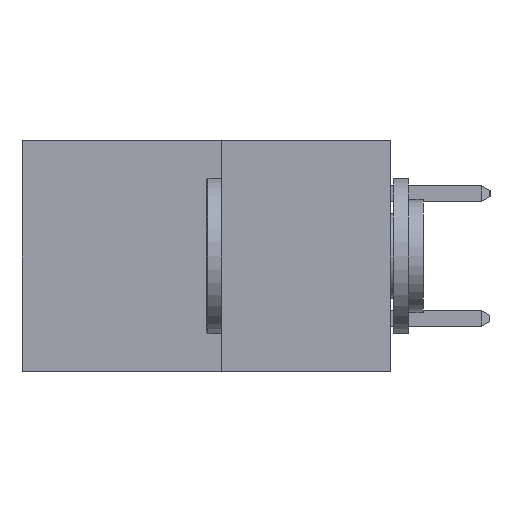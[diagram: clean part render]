
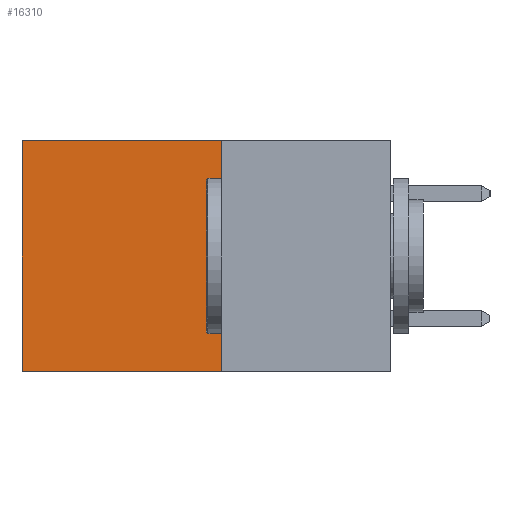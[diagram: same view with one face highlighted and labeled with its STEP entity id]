
A CAD part, left-side view. The second image highlights one B-rep face of the part: STEP entity #16310.
In plain terms, the highlighted planar face has unit normal (-1, 0, 0).
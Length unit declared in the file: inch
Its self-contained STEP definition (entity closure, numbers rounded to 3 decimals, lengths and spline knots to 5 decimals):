
#34 = ORIENTED_EDGE ( 'NONE', *, *, #13516, .T. ) ;
#1484 = LINE ( 'NONE', #3743, #8843 ) ;
#2045 = VECTOR ( 'NONE', #7457, 39.37008 ) ;
#2546 = CARTESIAN_POINT ( 'NONE',  ( 0.277, 0.27, -0.37 ) ) ;
#2694 = DIRECTION ( 'NONE',  ( 0., 0., -1. ) ) ;
#2804 = VERTEX_POINT ( 'NONE', #28095 ) ;
#2825 = DIRECTION ( 'NONE',  ( 0., 0., -1. ) ) ;
#3565 = VECTOR ( 'NONE', #2825, 39.37008 ) ;
#3742 = VERTEX_POINT ( 'NONE', #18496 ) ;
#3743 = CARTESIAN_POINT ( 'NONE',  ( 0.277, 0.27, 0. ) ) ;
#4369 = LINE ( 'NONE', #24317, #2045 ) ;
#5037 = DIRECTION ( 'NONE',  ( 0., 0., -1. ) ) ;
#6845 = AXIS2_PLACEMENT_3D ( 'NONE', #2546, #19517, #5037 ) ;
#7457 = DIRECTION ( 'NONE',  ( 0., 1., 0. ) ) ;
#7569 = CARTESIAN_POINT ( 'NONE',  ( 0.277, 0.27, -0.37 ) ) ;
#7700 = EDGE_CURVE ( 'NONE', #15759, #2804, #1484, .T. ) ;
#8843 = VECTOR ( 'NONE', #13394, 39.37008 ) ;
#9812 = PLANE ( 'NONE',  #6845 ) ;
#10057 = LINE ( 'NONE', #14929, #3565 ) ;
#10149 = EDGE_LOOP ( 'NONE', ( #34, #19327, #25335, #21019 ) ) ;
#11884 = EDGE_CURVE ( 'NONE', #15759, #24235, #10057, .T. ) ;
#13394 = DIRECTION ( 'NONE',  ( 0., 1., 0. ) ) ;
#13516 = EDGE_CURVE ( 'NONE', #2804, #3742, #28811, .T. ) ;
#14929 = CARTESIAN_POINT ( 'NONE',  ( 0.277, 0.27, -0.37 ) ) ;
#15759 = VERTEX_POINT ( 'NONE', #17684 ) ;
#16310 = ADVANCED_FACE ( 'NONE', ( #30087 ), #9812, .F. ) ;
#17684 = CARTESIAN_POINT ( 'NONE',  ( 0.277, 0.27, 0. ) ) ;
#18496 = CARTESIAN_POINT ( 'NONE',  ( 0.277, 0.59, -0.37 ) ) ;
#19327 = ORIENTED_EDGE ( 'NONE', *, *, #22319, .F. ) ;
#19517 = DIRECTION ( 'NONE',  ( 1., 0., 0. ) ) ;
#21019 = ORIENTED_EDGE ( 'NONE', *, *, #7700, .T. ) ;
#22319 = EDGE_CURVE ( 'NONE', #24235, #3742, #4369, .T. ) ;
#22466 = VECTOR ( 'NONE', #2694, 39.37008 ) ;
#24235 = VERTEX_POINT ( 'NONE', #7569 ) ;
#24317 = CARTESIAN_POINT ( 'NONE',  ( 0.277, 0.27, -0.37 ) ) ;
#24365 = CARTESIAN_POINT ( 'NONE',  ( 0.277, 0.59, -0.37 ) ) ;
#25335 = ORIENTED_EDGE ( 'NONE', *, *, #11884, .F. ) ;
#28095 = CARTESIAN_POINT ( 'NONE',  ( 0.277, 0.59, 0. ) ) ;
#28811 = LINE ( 'NONE', #24365, #22466 ) ;
#30087 = FACE_OUTER_BOUND ( 'NONE', #10149, .T. ) ;
